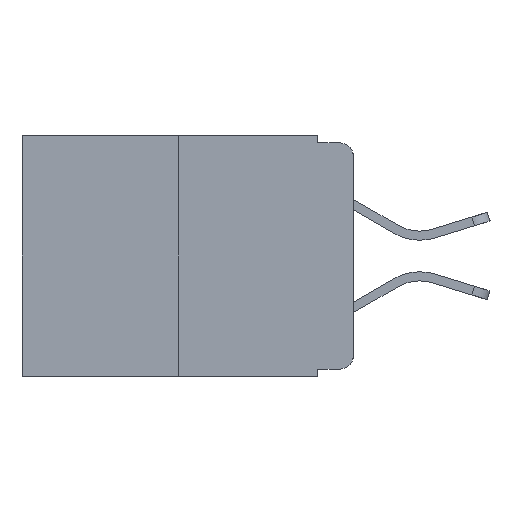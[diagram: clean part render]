
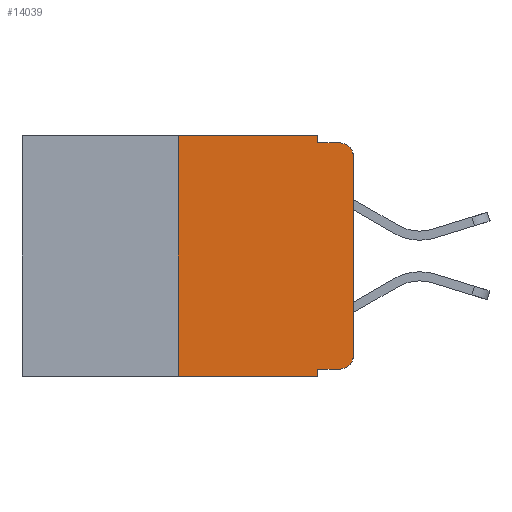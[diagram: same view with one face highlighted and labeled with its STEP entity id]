
A CAD part, left-side view. The second image highlights one B-rep face of the part: STEP entity #14039.
In plain terms, the highlighted planar face has unit normal (-1, 0, 0).
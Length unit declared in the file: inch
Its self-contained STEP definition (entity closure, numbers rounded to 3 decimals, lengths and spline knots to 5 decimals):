
#24 = CARTESIAN_POINT ( 'NONE',  ( 0., 0.051, 0. ) ) ;
#468 = DIRECTION ( 'NONE',  ( 0., -1., 0. ) ) ;
#610 = EDGE_CURVE ( 'NONE', #13059, #5159, #8261, .T. ) ;
#708 = VERTEX_POINT ( 'NONE', #6113 ) ;
#1090 = VERTEX_POINT ( 'NONE', #4998 ) ;
#1147 = DIRECTION ( 'NONE',  ( 0., -1., 0. ) ) ;
#1584 = CIRCLE ( 'NONE', #14747, 0.02 ) ;
#1631 = VERTEX_POINT ( 'NONE', #12360 ) ;
#1928 = ORIENTED_EDGE ( 'NONE', *, *, #7813, .F. ) ;
#1944 = VERTEX_POINT ( 'NONE', #6765 ) ;
#1983 = CARTESIAN_POINT ( 'NONE',  ( 0., 0.051, -0.01 ) ) ;
#2098 = CARTESIAN_POINT ( 'NONE',  ( 0., 0., 0. ) ) ;
#2232 = LINE ( 'NONE', #1983, #11009 ) ;
#2249 = EDGE_CURVE ( 'NONE', #6989, #708, #8039, .T. ) ;
#2260 = CARTESIAN_POINT ( 'NONE',  ( 0., 0.02, -0.01 ) ) ;
#2293 = VECTOR ( 'NONE', #468, 39.37008 ) ;
#2477 = EDGE_LOOP ( 'NONE', ( #5254, #5617, #2829, #12644, #1928, #3384, #10565, #5268, #8794, #13499 ) ) ;
#2690 = VECTOR ( 'NONE', #1147, 39.37008 ) ;
#2786 = VECTOR ( 'NONE', #7269, 39.37008 ) ;
#2829 = ORIENTED_EDGE ( 'NONE', *, *, #5417, .F. ) ;
#2843 = CARTESIAN_POINT ( 'NONE',  ( 0., 0.473, -0.343 ) ) ;
#2876 = DIRECTION ( 'NONE',  ( 0., -1., 0. ) ) ;
#3158 = LINE ( 'NONE', #24, #2786 ) ;
#3304 = EDGE_CURVE ( 'NONE', #1090, #4889, #10105, .T. ) ;
#3384 = ORIENTED_EDGE ( 'NONE', *, *, #2249, .F. ) ;
#3425 = DIRECTION ( 'NONE',  ( 0., 0., 1. ) ) ;
#3560 = DIRECTION ( 'NONE',  ( 0., 0., -1. ) ) ;
#3685 = CARTESIAN_POINT ( 'NONE',  ( 0., 0.25, 0. ) ) ;
#4397 = DIRECTION ( 'NONE',  ( 0., 0., -1. ) ) ;
#4633 = EDGE_CURVE ( 'NONE', #1631, #1944, #3158, .T. ) ;
#4889 = VERTEX_POINT ( 'NONE', #5806 ) ;
#4998 = CARTESIAN_POINT ( 'NONE',  ( 0., 0.02, -0.333 ) ) ;
#5126 = LINE ( 'NONE', #9267, #2690 ) ;
#5159 = VERTEX_POINT ( 'NONE', #14543 ) ;
#5254 = ORIENTED_EDGE ( 'NONE', *, *, #11453, .T. ) ;
#5268 = ORIENTED_EDGE ( 'NONE', *, *, #610, .F. ) ;
#5417 = EDGE_CURVE ( 'NONE', #1944, #6872, #2232, .T. ) ;
#5479 = AXIS2_PLACEMENT_3D ( 'NONE', #8962, #11203, #4397 ) ;
#5490 = LINE ( 'NONE', #2098, #11122 ) ;
#5617 = ORIENTED_EDGE ( 'NONE', *, *, #8471, .T. ) ;
#5790 = LINE ( 'NONE', #2843, #2293 ) ;
#5806 = CARTESIAN_POINT ( 'NONE',  ( 0., 0., -0.313 ) ) ;
#5881 = DIRECTION ( 'NONE',  ( -1., 0., 0. ) ) ;
#6113 = CARTESIAN_POINT ( 'NONE',  ( 0., 0.25, 0. ) ) ;
#6197 = CARTESIAN_POINT ( 'NONE',  ( 0., 0.051, -0.333 ) ) ;
#6199 = CARTESIAN_POINT ( 'NONE',  ( 0., 0.25, -0.343 ) ) ;
#6310 = FACE_OUTER_BOUND ( 'NONE', #2477, .T. ) ;
#6765 = CARTESIAN_POINT ( 'NONE',  ( 0., 0.051, -0.01 ) ) ;
#6872 = VERTEX_POINT ( 'NONE', #2260 ) ;
#6972 = DIRECTION ( 'NONE',  ( 0., 0., -1. ) ) ;
#6987 = DIRECTION ( 'NONE',  ( -1., 0., 0. ) ) ;
#6989 = VERTEX_POINT ( 'NONE', #6199 ) ;
#7269 = DIRECTION ( 'NONE',  ( 0., 0., -1. ) ) ;
#7813 = EDGE_CURVE ( 'NONE', #708, #1631, #5126, .T. ) ;
#8039 = LINE ( 'NONE', #3685, #10655 ) ;
#8102 = CARTESIAN_POINT ( 'NONE',  ( 0., 0.051, 0. ) ) ;
#8261 = LINE ( 'NONE', #8102, #11571 ) ;
#8306 = VECTOR ( 'NONE', #2876, 39.37008 ) ;
#8471 = EDGE_CURVE ( 'NONE', #14512, #6872, #1584, .T. ) ;
#8652 = CARTESIAN_POINT ( 'NONE',  ( 0., 0.051, -0.333 ) ) ;
#8794 = ORIENTED_EDGE ( 'NONE', *, *, #12473, .T. ) ;
#8910 = PLANE ( 'NONE',  #5479 ) ;
#8962 = CARTESIAN_POINT ( 'NONE',  ( 0., 0.473, 0. ) ) ;
#9267 = CARTESIAN_POINT ( 'NONE',  ( 0., 0.473, 0. ) ) ;
#10105 = CIRCLE ( 'NONE', #14783, 0.02 ) ;
#10565 = ORIENTED_EDGE ( 'NONE', *, *, #13841, .T. ) ;
#10655 = VECTOR ( 'NONE', #3425, 39.37008 ) ;
#11009 = VECTOR ( 'NONE', #12444, 39.37008 ) ;
#11122 = VECTOR ( 'NONE', #13466, 39.37008 ) ;
#11203 = DIRECTION ( 'NONE',  ( 1., 0., 0. ) ) ;
#11270 = LINE ( 'NONE', #8652, #8306 ) ;
#11453 = EDGE_CURVE ( 'NONE', #4889, #14512, #5490, .T. ) ;
#11571 = VECTOR ( 'NONE', #3560, 39.37008 ) ;
#12360 = CARTESIAN_POINT ( 'NONE',  ( 0., 0.051, 0. ) ) ;
#12444 = DIRECTION ( 'NONE',  ( 0., -1., 0. ) ) ;
#12473 = EDGE_CURVE ( 'NONE', #13059, #1090, #11270, .T. ) ;
#12529 = CARTESIAN_POINT ( 'NONE',  ( 0., 0.02, -0.313 ) ) ;
#12600 = CARTESIAN_POINT ( 'NONE',  ( 0., 0.02, -0.03 ) ) ;
#12644 = ORIENTED_EDGE ( 'NONE', *, *, #4633, .F. ) ;
#13059 = VERTEX_POINT ( 'NONE', #6197 ) ;
#13466 = DIRECTION ( 'NONE',  ( 0., 0., 1. ) ) ;
#13499 = ORIENTED_EDGE ( 'NONE', *, *, #3304, .T. ) ;
#13676 = DIRECTION ( 'NONE',  ( 0., 0., -1. ) ) ;
#13841 = EDGE_CURVE ( 'NONE', #6989, #5159, #5790, .T. ) ;
#14039 = ADVANCED_FACE ( 'NONE', ( #6310 ), #8910, .F. ) ;
#14313 = CARTESIAN_POINT ( 'NONE',  ( 0., 0., -0.03 ) ) ;
#14512 = VERTEX_POINT ( 'NONE', #14313 ) ;
#14543 = CARTESIAN_POINT ( 'NONE',  ( 0., 0.051, -0.343 ) ) ;
#14747 = AXIS2_PLACEMENT_3D ( 'NONE', #12600, #5881, #13676 ) ;
#14783 = AXIS2_PLACEMENT_3D ( 'NONE', #12529, #6987, #6972 ) ;
